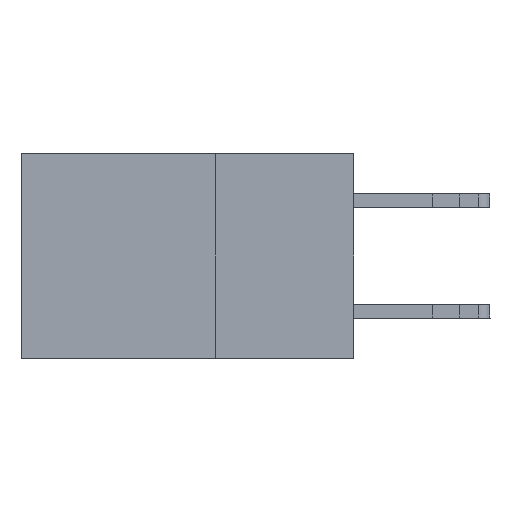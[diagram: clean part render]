
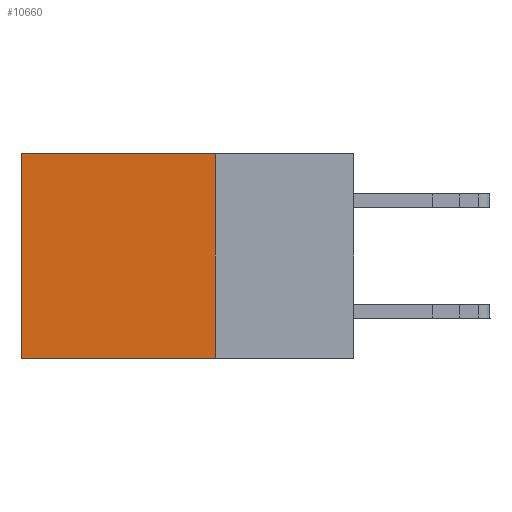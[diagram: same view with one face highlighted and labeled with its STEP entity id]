
A CAD part, left-side view. The second image highlights one B-rep face of the part: STEP entity #10660.
In plain terms, the highlighted planar face has unit normal (-1, 0, 0).
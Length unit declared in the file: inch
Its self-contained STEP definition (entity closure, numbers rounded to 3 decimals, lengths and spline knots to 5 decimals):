
#817 = LINE ( 'NONE', #17218, #13795 ) ;
#905 = CARTESIAN_POINT ( 'NONE',  ( 0.2875, 0.25, 0. ) ) ;
#1274 = LINE ( 'NONE', #3563, #14319 ) ;
#1276 = LINE ( 'NONE', #8194, #12016 ) ;
#2298 = VERTEX_POINT ( 'NONE', #9909 ) ;
#3192 = ORIENTED_EDGE ( 'NONE', *, *, #11596, .T. ) ;
#3287 = ORIENTED_EDGE ( 'NONE', *, *, #3746, .T. ) ;
#3563 = CARTESIAN_POINT ( 'NONE',  ( 0.2875, 0.6, 0. ) ) ;
#3746 = EDGE_CURVE ( 'NONE', #12279, #11556, #13095, .T. ) ;
#4089 = ORIENTED_EDGE ( 'NONE', *, *, #15263, .F. ) ;
#4664 = CARTESIAN_POINT ( 'NONE',  ( 0.2875, 0.25, 0. ) ) ;
#4947 = DIRECTION ( 'NONE',  ( 0., 1., 0. ) ) ;
#5778 = CARTESIAN_POINT ( 'NONE',  ( 0.2875, 0.25, 0. ) ) ;
#6020 = EDGE_LOOP ( 'NONE', ( #3192, #4089, #11956, #3287 ) ) ;
#6191 = DIRECTION ( 'NONE',  ( 0., 1., 0. ) ) ;
#6330 = DIRECTION ( 'NONE',  ( 0., 0., -1. ) ) ;
#6744 = DIRECTION ( 'NONE',  ( 0., 0., -1. ) ) ;
#7070 = VECTOR ( 'NONE', #6191, 39.37008 ) ;
#7484 = PLANE ( 'NONE',  #10559 ) ;
#8194 = CARTESIAN_POINT ( 'NONE',  ( 0.2875, 0.25, 0. ) ) ;
#8433 = VERTEX_POINT ( 'NONE', #14330 ) ;
#9909 = CARTESIAN_POINT ( 'NONE',  ( 0.2875, 0.25, -0.37 ) ) ;
#10559 = AXIS2_PLACEMENT_3D ( 'NONE', #5778, #12690, #14380 ) ;
#10660 = ADVANCED_FACE ( 'NONE', ( #12770 ), #7484, .F. ) ;
#11556 = VERTEX_POINT ( 'NONE', #13659 ) ;
#11596 = EDGE_CURVE ( 'NONE', #11556, #8433, #1274, .T. ) ;
#11956 = ORIENTED_EDGE ( 'NONE', *, *, #13536, .F. ) ;
#12016 = VECTOR ( 'NONE', #6744, 39.37008 ) ;
#12279 = VERTEX_POINT ( 'NONE', #4664 ) ;
#12690 = DIRECTION ( 'NONE',  ( 1., 0., 0. ) ) ;
#12770 = FACE_OUTER_BOUND ( 'NONE', #6020, .T. ) ;
#13095 = LINE ( 'NONE', #905, #7070 ) ;
#13536 = EDGE_CURVE ( 'NONE', #12279, #2298, #1276, .T. ) ;
#13659 = CARTESIAN_POINT ( 'NONE',  ( 0.2875, 0.6, 0. ) ) ;
#13795 = VECTOR ( 'NONE', #4947, 39.37008 ) ;
#14319 = VECTOR ( 'NONE', #6330, 39.37008 ) ;
#14330 = CARTESIAN_POINT ( 'NONE',  ( 0.2875, 0.6, -0.37 ) ) ;
#14380 = DIRECTION ( 'NONE',  ( 0., 0., -1. ) ) ;
#15263 = EDGE_CURVE ( 'NONE', #2298, #8433, #817, .T. ) ;
#17218 = CARTESIAN_POINT ( 'NONE',  ( 0.2875, 0.25, -0.37 ) ) ;
